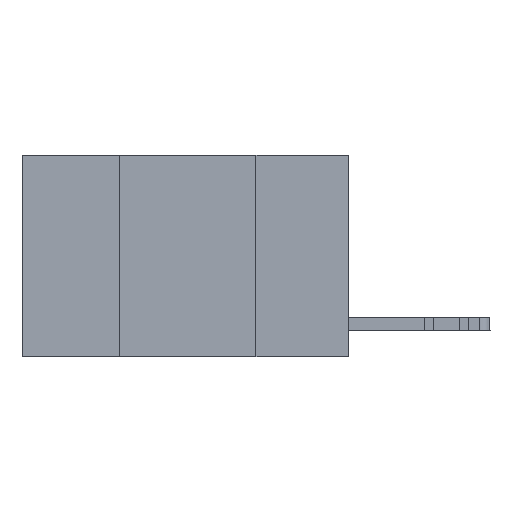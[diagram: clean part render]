
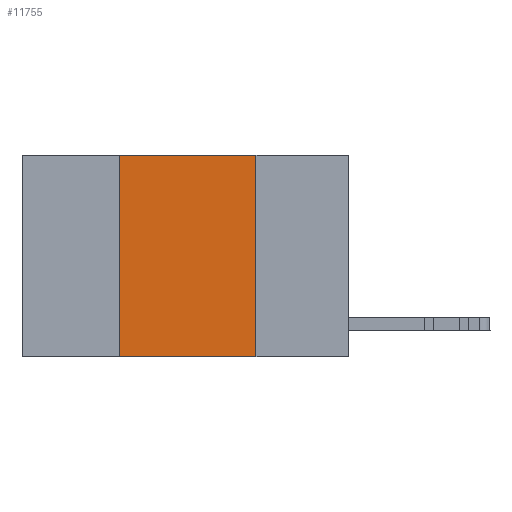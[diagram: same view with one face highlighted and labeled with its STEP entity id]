
A CAD part, left-side view. The second image highlights one B-rep face of the part: STEP entity #11755.
In plain terms, the highlighted planar face has unit normal (-1, 0, 0).
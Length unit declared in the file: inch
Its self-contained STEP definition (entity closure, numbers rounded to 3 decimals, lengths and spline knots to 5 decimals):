
#983 = CARTESIAN_POINT ( 'NONE',  ( 0., 0.42, 0. ) ) ;
#2049 = LINE ( 'NONE', #17025, #16696 ) ;
#2680 = EDGE_CURVE ( 'NONE', #21648, #20249, #28198, .T. ) ;
#3114 = LINE ( 'NONE', #14328, #19432 ) ;
#3157 = EDGE_CURVE ( 'NONE', #20249, #16474, #3114, .T. ) ;
#3788 = DIRECTION ( 'NONE',  ( 0., -1., 0. ) ) ;
#4775 = DIRECTION ( 'NONE',  ( 0., 0., -1. ) ) ;
#5166 = CARTESIAN_POINT ( 'NONE',  ( 0., 0.17, -0.37 ) ) ;
#9204 = DIRECTION ( 'NONE',  ( 0., 0., -1. ) ) ;
#9469 = VECTOR ( 'NONE', #14357, 39.37008 ) ;
#10090 = DIRECTION ( 'NONE',  ( 0., -1., 0. ) ) ;
#11755 = ADVANCED_FACE ( 'NONE', ( #18002 ), #26738, .F. ) ;
#11847 = EDGE_LOOP ( 'NONE', ( #20952, #14820, #23804, #25544 ) ) ;
#14328 = CARTESIAN_POINT ( 'NONE',  ( 0., 0.6, 0. ) ) ;
#14357 = DIRECTION ( 'NONE',  ( 0., 0., 1. ) ) ;
#14820 = ORIENTED_EDGE ( 'NONE', *, *, #3157, .F. ) ;
#15831 = LINE ( 'NONE', #20803, #25166 ) ;
#16229 = DIRECTION ( 'NONE',  ( 1., 0., 0. ) ) ;
#16474 = VERTEX_POINT ( 'NONE', #28001 ) ;
#16696 = VECTOR ( 'NONE', #3788, 39.37008 ) ;
#17025 = CARTESIAN_POINT ( 'NONE',  ( 0., 0.6, -0.37 ) ) ;
#18002 = FACE_OUTER_BOUND ( 'NONE', #11847, .T. ) ;
#18397 = EDGE_CURVE ( 'NONE', #16474, #20173, #15831, .T. ) ;
#19432 = VECTOR ( 'NONE', #10090, 39.37008 ) ;
#20173 = VERTEX_POINT ( 'NONE', #5166 ) ;
#20249 = VERTEX_POINT ( 'NONE', #23088 ) ;
#20700 = EDGE_CURVE ( 'NONE', #21648, #20173, #2049, .T. ) ;
#20803 = CARTESIAN_POINT ( 'NONE',  ( 0., 0.17, 0. ) ) ;
#20952 = ORIENTED_EDGE ( 'NONE', *, *, #18397, .F. ) ;
#21648 = VERTEX_POINT ( 'NONE', #26142 ) ;
#23088 = CARTESIAN_POINT ( 'NONE',  ( 0., 0.42, 0. ) ) ;
#23804 = ORIENTED_EDGE ( 'NONE', *, *, #2680, .F. ) ;
#25166 = VECTOR ( 'NONE', #4775, 39.37008 ) ;
#25544 = ORIENTED_EDGE ( 'NONE', *, *, #20700, .T. ) ;
#26142 = CARTESIAN_POINT ( 'NONE',  ( 0., 0.42, -0.37 ) ) ;
#26358 = AXIS2_PLACEMENT_3D ( 'NONE', #26883, #16229, #9204 ) ;
#26738 = PLANE ( 'NONE',  #26358 ) ;
#26883 = CARTESIAN_POINT ( 'NONE',  ( 0., 0.6, 0. ) ) ;
#28001 = CARTESIAN_POINT ( 'NONE',  ( 0., 0.17, 0. ) ) ;
#28198 = LINE ( 'NONE', #983, #9469 ) ;
